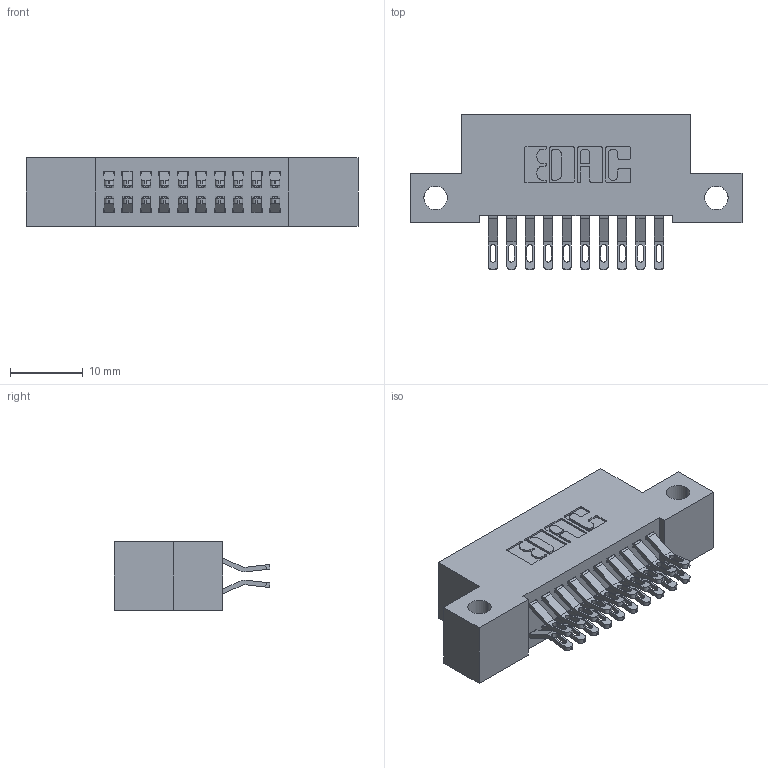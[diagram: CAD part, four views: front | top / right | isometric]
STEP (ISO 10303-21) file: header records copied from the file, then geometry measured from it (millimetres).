
FILE_DESCRIPTION (( 'STEP AP203' ), '1' );
FILE_NAME ('342-020-555-212.STEP', '2018-08-10T23:16:37', ( '' ), ( '' ), 'SwSTEP 2.0', 'SolidWorks 2016', '' );
FILE_SCHEMA (( 'CONFIG_CONTROL_DESIGN' ));
Length unit declared in the file: inch
Products named in the file (3): 342 Part_Side Mount; 345-292-001_555 Tail; 342-020-555-212
Assembly tree (21 placements, depth 2):
  342-020-555-212
    342 Part_Side Mount
    345-292-001_555 Tail  x20
Bounding box: 45.72 x 21.47 x 9.4 mm (x, y, z)
Volume: 3938.1 mm3; surface area: 5655.5 mm2
Topology: 21 solids, 21 shells, 1270 faces, 3959 edges, 2638 vertices
Faces by surface type: plane 746, cylinder 524
Entity records: 10769 total; most frequent: CARTESIAN_POINT 1856, ORIENTED_EDGE 1762, DIRECTION 1613, EDGE_CURVE 881, LINE 733, VECTOR 733, VERTEX_POINT 586, AXIS2_PLACEMENT_3D 440
